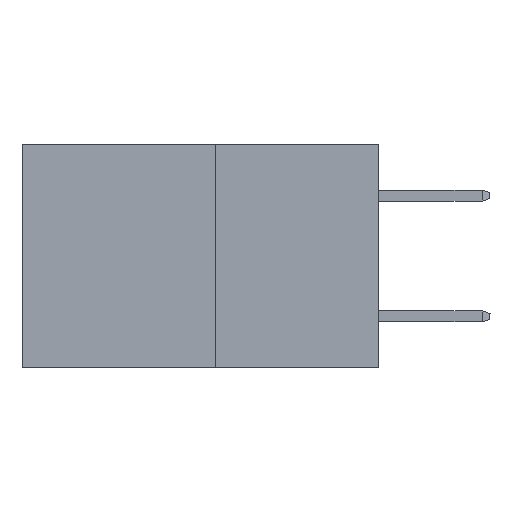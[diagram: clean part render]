
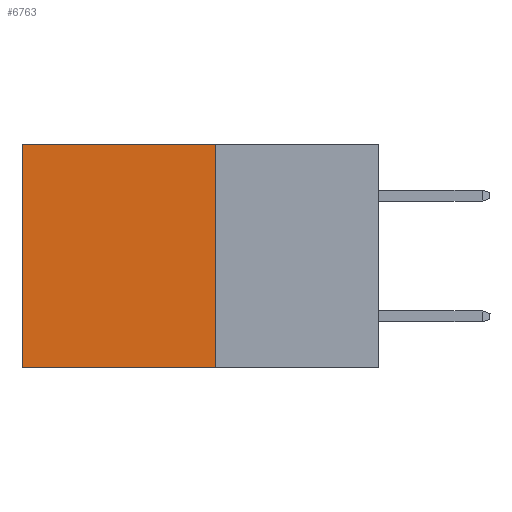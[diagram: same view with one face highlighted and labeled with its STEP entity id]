
A CAD part, left-side view. The second image highlights one B-rep face of the part: STEP entity #6763.
In plain terms, the highlighted planar face has unit normal (-1, 0, 0).
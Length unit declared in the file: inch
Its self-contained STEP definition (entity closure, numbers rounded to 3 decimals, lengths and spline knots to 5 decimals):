
#105 = DIRECTION ( 'NONE',  ( 0., 1., 0. ) ) ;
#715 = AXIS2_PLACEMENT_3D ( 'NONE', #4417, #4400, #4366 ) ;
#2114 = ORIENTED_EDGE ( 'NONE', *, *, #14628, .T. ) ;
#2549 = ORIENTED_EDGE ( 'NONE', *, *, #15921, .F. ) ;
#2668 = CARTESIAN_POINT ( 'NONE',  ( 0.277, 0.27, -0.37 ) ) ;
#2717 = EDGE_CURVE ( 'NONE', #2869, #15893, #4487, .T. ) ;
#2742 = ORIENTED_EDGE ( 'NONE', *, *, #10353, .F. ) ;
#2869 = VERTEX_POINT ( 'NONE', #13229 ) ;
#2932 = DIRECTION ( 'NONE',  ( 0., 0., -1. ) ) ;
#2957 = VECTOR ( 'NONE', #10724, 39.37008 ) ;
#3385 = LINE ( 'NONE', #2668, #2957 ) ;
#3749 = ORIENTED_EDGE ( 'NONE', *, *, #2717, .T. ) ;
#4366 = DIRECTION ( 'NONE',  ( 0., 0., -1. ) ) ;
#4400 = DIRECTION ( 'NONE',  ( 1., 0., 0. ) ) ;
#4417 = CARTESIAN_POINT ( 'NONE',  ( 0.277, 0.27, -0.37 ) ) ;
#4487 = LINE ( 'NONE', #6240, #11240 ) ;
#4541 = PLANE ( 'NONE',  #715 ) ;
#4817 = EDGE_LOOP ( 'NONE', ( #2114, #2549, #2742, #3749 ) ) ;
#5150 = CARTESIAN_POINT ( 'NONE',  ( 0.277, 0.27, -0.37 ) ) ;
#5803 = VECTOR ( 'NONE', #105, 39.37008 ) ;
#6240 = CARTESIAN_POINT ( 'NONE',  ( 0.277, 0.27, 0. ) ) ;
#6421 = LINE ( 'NONE', #9681, #9601 ) ;
#6735 = VERTEX_POINT ( 'NONE', #5150 ) ;
#6763 = ADVANCED_FACE ( 'NONE', ( #15404 ), #4541, .F. ) ;
#6795 = CARTESIAN_POINT ( 'NONE',  ( 0.277, 0.59, 0. ) ) ;
#6866 = DIRECTION ( 'NONE',  ( 0., 1., 0. ) ) ;
#8231 = CARTESIAN_POINT ( 'NONE',  ( 0.277, 0.27, -0.37 ) ) ;
#9601 = VECTOR ( 'NONE', #2932, 39.37008 ) ;
#9681 = CARTESIAN_POINT ( 'NONE',  ( 0.277, 0.59, -0.37 ) ) ;
#10353 = EDGE_CURVE ( 'NONE', #2869, #6735, #3385, .T. ) ;
#10724 = DIRECTION ( 'NONE',  ( 0., 0., -1. ) ) ;
#11240 = VECTOR ( 'NONE', #6866, 39.37008 ) ;
#13229 = CARTESIAN_POINT ( 'NONE',  ( 0.277, 0.27, 0. ) ) ;
#13928 = CARTESIAN_POINT ( 'NONE',  ( 0.277, 0.59, -0.37 ) ) ;
#14628 = EDGE_CURVE ( 'NONE', #15893, #14788, #6421, .T. ) ;
#14788 = VERTEX_POINT ( 'NONE', #13928 ) ;
#15404 = FACE_OUTER_BOUND ( 'NONE', #4817, .T. ) ;
#15893 = VERTEX_POINT ( 'NONE', #6795 ) ;
#15921 = EDGE_CURVE ( 'NONE', #6735, #14788, #16798, .T. ) ;
#16798 = LINE ( 'NONE', #8231, #5803 ) ;
